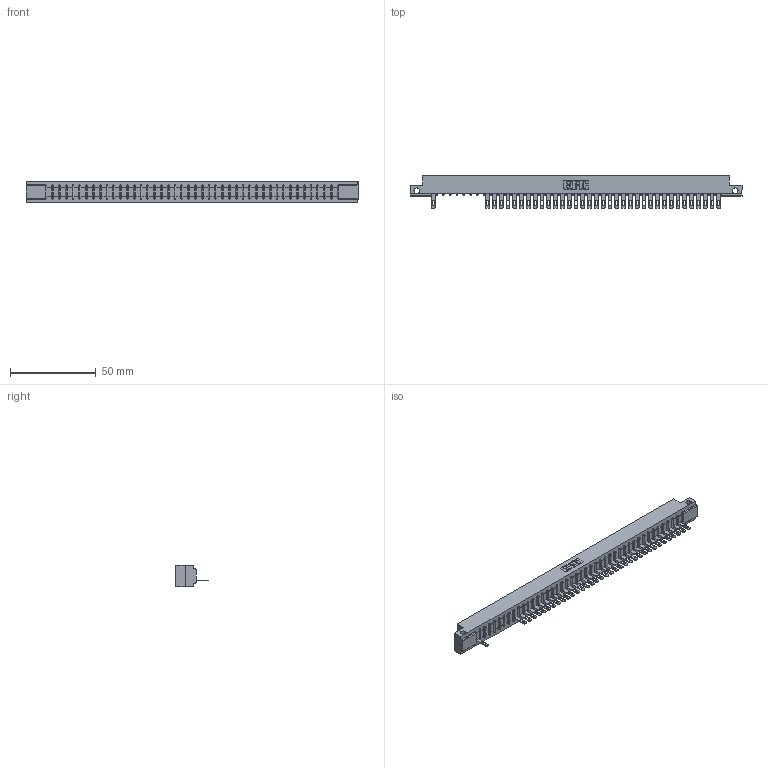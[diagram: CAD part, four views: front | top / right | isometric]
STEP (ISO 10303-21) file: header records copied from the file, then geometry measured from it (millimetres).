
FILE_DESCRIPTION (( 'STEP AP203' ), '1' );
FILE_NAME ('307-043-505-112.STEP', '2018-08-05T18:51:18', ( '' ), ( '' ), 'SwSTEP 2.0', 'SolidWorks 2016', '' );
FILE_SCHEMA (( 'CONFIG_CONTROL_DESIGN' ));
Length unit declared in the file: inch
Products named in the file (3): 307-290-001_505; 307-043-505-112; 307 Part_.128 Dia Side Mounting Holes
Assembly tree (37 placements, depth 2):
  307-043-505-112
    307 Part_.128 Dia Side Mounting Holes
    307-290-001_505  x36
Bounding box: 193.4 x 19.18 x 12.7 mm (x, y, z)
Volume: 19887.7 mm3; surface area: 20672.9 mm2
Topology: 37 solids, 37 shells, 2318 faces, 6603 edges, 4234 vertices
Faces by surface type: plane 1450, cylinder 780, sphere 88
Entity records: 36492 total; most frequent: CARTESIAN_POINT 6177, ORIENTED_EDGE 6170, DIRECTION 6001, EDGE_CURVE 3085, LINE 2365, VECTOR 2365, VERTEX_POINT 1994, AXIS2_PLACEMENT_3D 1818
